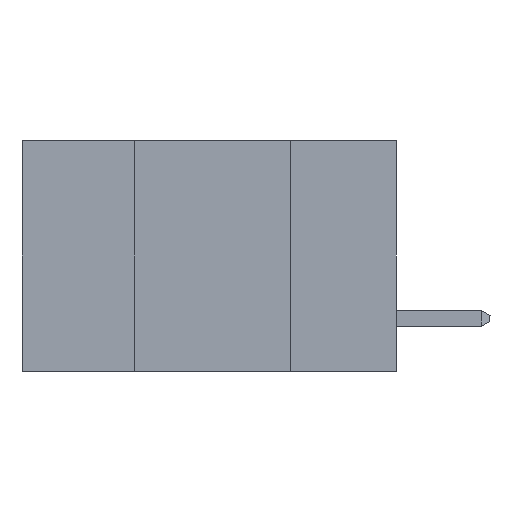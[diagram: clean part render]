
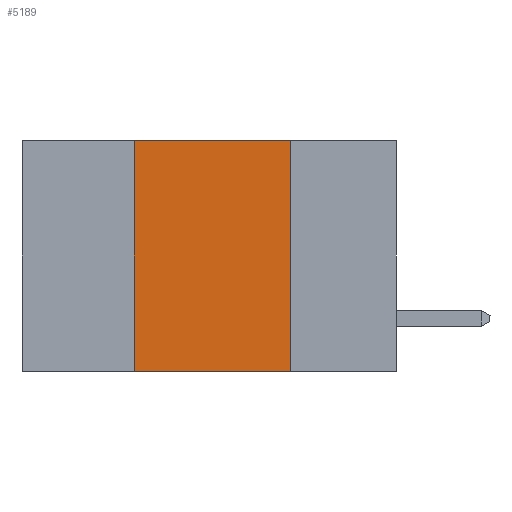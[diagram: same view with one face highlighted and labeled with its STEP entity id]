
A CAD part, left-side view. The second image highlights one B-rep face of the part: STEP entity #5189.
In plain terms, the highlighted planar face has unit normal (-1, 0, 0).
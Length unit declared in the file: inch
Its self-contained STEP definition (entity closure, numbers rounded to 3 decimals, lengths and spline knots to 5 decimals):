
#827 = VECTOR ( 'NONE', #14810, 39.37008 ) ;
#1601 = CARTESIAN_POINT ( 'NONE',  ( 0., 0.42, 0. ) ) ;
#1908 = EDGE_CURVE ( 'NONE', #22121, #6852, #13281, .T. ) ;
#3543 = VECTOR ( 'NONE', #15014, 39.37008 ) ;
#4443 = EDGE_CURVE ( 'NONE', #6852, #13400, #9656, .T. ) ;
#5189 = ADVANCED_FACE ( 'NONE', ( #5256 ), #13876, .F. ) ;
#5256 = FACE_OUTER_BOUND ( 'NONE', #20564, .T. ) ;
#6115 = DIRECTION ( 'NONE',  ( 0., 0., -1. ) ) ;
#6852 = VERTEX_POINT ( 'NONE', #20919 ) ;
#8832 = DIRECTION ( 'NONE',  ( 1., 0., 0. ) ) ;
#9656 = LINE ( 'NONE', #21470, #16944 ) ;
#10657 = ORIENTED_EDGE ( 'NONE', *, *, #21080, .T. ) ;
#10962 = ORIENTED_EDGE ( 'NONE', *, *, #1908, .F. ) ;
#11097 = EDGE_CURVE ( 'NONE', #20334, #22121, #21898, .T. ) ;
#11490 = LINE ( 'NONE', #14837, #15557 ) ;
#11540 = CARTESIAN_POINT ( 'NONE',  ( 0., 0.17, -0.37 ) ) ;
#12251 = CARTESIAN_POINT ( 'NONE',  ( 0., 0.6, 0. ) ) ;
#13281 = LINE ( 'NONE', #20044, #3543 ) ;
#13400 = VERTEX_POINT ( 'NONE', #11540 ) ;
#13876 = PLANE ( 'NONE',  #14268 ) ;
#14268 = AXIS2_PLACEMENT_3D ( 'NONE', #12251, #8832, #17507 ) ;
#14810 = DIRECTION ( 'NONE',  ( 0., 0., 1. ) ) ;
#14837 = CARTESIAN_POINT ( 'NONE',  ( 0., 0.6, -0.37 ) ) ;
#15014 = DIRECTION ( 'NONE',  ( 0., -1., 0. ) ) ;
#15557 = VECTOR ( 'NONE', #18015, 39.37008 ) ;
#15705 = ORIENTED_EDGE ( 'NONE', *, *, #11097, .F. ) ;
#16944 = VECTOR ( 'NONE', #6115, 39.37008 ) ;
#17507 = DIRECTION ( 'NONE',  ( 0., 0., -1. ) ) ;
#17980 = ORIENTED_EDGE ( 'NONE', *, *, #4443, .F. ) ;
#18015 = DIRECTION ( 'NONE',  ( 0., -1., 0. ) ) ;
#20044 = CARTESIAN_POINT ( 'NONE',  ( 0., 0.6, 0. ) ) ;
#20334 = VERTEX_POINT ( 'NONE', #21561 ) ;
#20564 = EDGE_LOOP ( 'NONE', ( #17980, #10962, #15705, #10657 ) ) ;
#20919 = CARTESIAN_POINT ( 'NONE',  ( 0., 0.17, 0. ) ) ;
#21080 = EDGE_CURVE ( 'NONE', #20334, #13400, #11490, .T. ) ;
#21470 = CARTESIAN_POINT ( 'NONE',  ( 0., 0.17, -0.37 ) ) ;
#21561 = CARTESIAN_POINT ( 'NONE',  ( 0., 0.42, -0.37 ) ) ;
#21785 = CARTESIAN_POINT ( 'NONE',  ( 0., 0.42, -0.37 ) ) ;
#21898 = LINE ( 'NONE', #21785, #827 ) ;
#22121 = VERTEX_POINT ( 'NONE', #1601 ) ;
